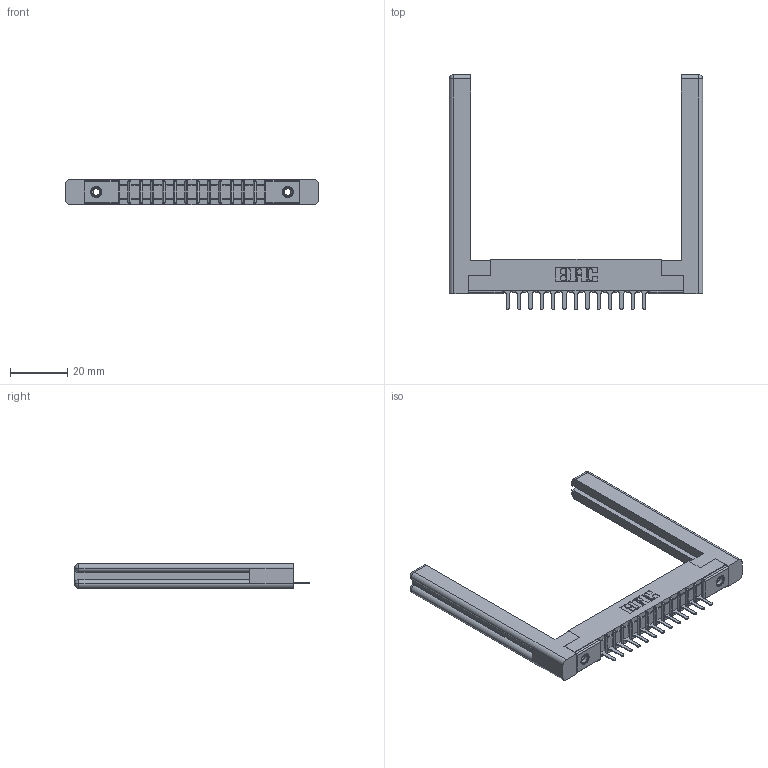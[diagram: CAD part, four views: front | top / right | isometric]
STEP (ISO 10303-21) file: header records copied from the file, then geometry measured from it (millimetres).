
FILE_DESCRIPTION (( 'STEP AP203' ), '1' );
FILE_NAME ('357-013-525-158.STEP', '2019-09-13T20:09:02', ( '' ), ( '' ), 'SwSTEP 2.0', 'SolidWorks 2016', '' );
FILE_SCHEMA (( 'CONFIG_CONTROL_DESIGN' ));
Length unit declared in the file: inch
Products named in the file (5): 307 Part_.156 Dia Mounting Holes; 345-250-001_345-250-001-102; 357-013-525-158; 307-290-001_525; 307-220-058
Assembly tree (18 placements, depth 2):
  357-013-525-158
    307 Part_.156 Dia Mounting Holes
    307-290-001_525  x13
    307-220-058  x2
    345-250-001_345-250-001-102  x2
Bounding box: 88.14 x 81.74 x 8.71 mm (x, y, z)
Volume: 13294.6 mm3; surface area: 13570.8 mm2
Topology: 18 solids, 18 shells, 1002 faces, 2783 edges, 1786 vertices
Faces by surface type: plane 635, cylinder 315, sphere 28, torus 12, cone 12
Entity records: 17321 total; most frequent: CARTESIAN_POINT 2915, ORIENTED_EDGE 2840, DIRECTION 2812, EDGE_CURVE 1420, LINE 1074, VECTOR 1074, VERTEX_POINT 918, AXIS2_PLACEMENT_3D 869
